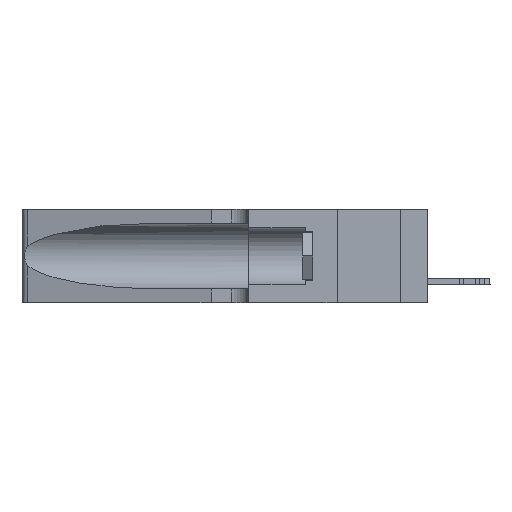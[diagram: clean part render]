
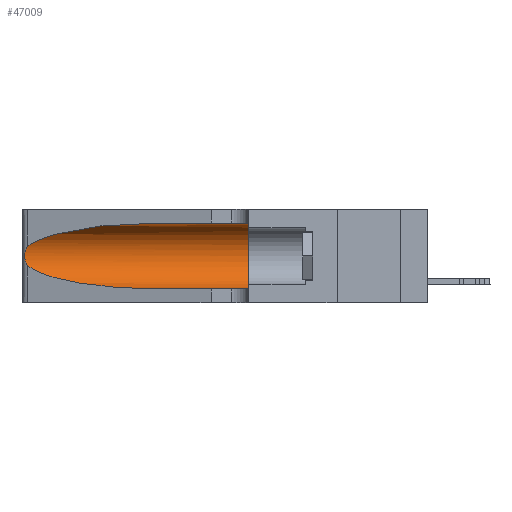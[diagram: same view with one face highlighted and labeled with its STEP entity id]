
A CAD part, left-side view. The second image highlights one B-rep face of the part: STEP entity #47009.
In plain terms, the highlighted cylindrical face has radius 3.308 mm (diameter 6.617 mm), a partial arc.
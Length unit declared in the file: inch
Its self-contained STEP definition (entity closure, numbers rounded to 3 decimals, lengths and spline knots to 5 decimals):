
#547 =( BOUNDED_CURVE ( )  B_SPLINE_CURVE ( 3, ( #36290, #44357, #9405, #29074 ),
 .UNSPECIFIED., .F., .F. ) 
 B_SPLINE_CURVE_WITH_KNOTS ( ( 4, 4 ),
 ( 3.44316, 4.71239 ),
 .UNSPECIFIED. ) 
 CURVE ( )  GEOMETRIC_REPRESENTATION_ITEM ( )  RATIONAL_B_SPLINE_CURVE ( ( 1., 0.87, 0.87, 1. ) ) 
 REPRESENTATION_ITEM ( '' )  );
#750 = EDGE_CURVE ( 'NONE', #4410, #35039, #23873, .T. ) ;
#972 = CARTESIAN_POINT ( 'NONE',  ( 0.25854, 1.2359, 0.20912 ) ) ;
#2075 = CARTESIAN_POINT ( 'NONE',  ( 0.1305, 0.35, 0.185 ) ) ;
#2380 = CARTESIAN_POINT ( 'NONE',  ( 0.25789, 1.23486, 0.15765 ) ) ;
#2528 = EDGE_CURVE ( 'NONE', #36630, #14953, #547, .T. ) ;
#3519 = AXIS2_PLACEMENT_3D ( 'NONE', #8318, #39538, #27631 ) ;
#3695 = LINE ( 'NONE', #27239, #42294 ) ;
#4410 = VERTEX_POINT ( 'NONE', #26532 ) ;
#4888 = CARTESIAN_POINT ( 'NONE',  ( 0.26018, 1.23835, 0.19895 ) ) ;
#4955 = ORIENTED_EDGE ( 'NONE', *, *, #2528, .T. ) ;
#5592 = CARTESIAN_POINT ( 'NONE',  ( 0.25487, 1.22718, 0.14631 ) ) ;
#5952 = CARTESIAN_POINT ( 'NONE',  ( 0.26017, 1.23833, 0.17102 ) ) ;
#7450 = LINE ( 'NONE', #18264, #44226 ) ;
#8318 = CARTESIAN_POINT ( 'NONE',  ( 0.1305, 1.61858, 0.185 ) ) ;
#8747 = CARTESIAN_POINT ( 'NONE',  ( 0.1305, 0.35, 0.05475 ) ) ;
#9405 = CARTESIAN_POINT ( 'NONE',  ( 0.18966, 0.96281, 0.05475 ) ) ;
#10429 = CARTESIAN_POINT ( 'NONE',  ( 0.25487, 1.22718, 0.14631 ) ) ;
#14953 = VERTEX_POINT ( 'NONE', #29104 ) ;
#16022 = ORIENTED_EDGE ( 'NONE', *, *, #750, .T. ) ;
#16343 = CARTESIAN_POINT ( 'NONE',  ( 0.25555, 1.22994, 0.2215 ) ) ;
#16745 = CARTESIAN_POINT ( 'NONE',  ( 0.2373, 1.15595, 0.28018 ) ) ;
#17580 = CARTESIAN_POINT ( 'NONE',  ( 0.1305, 0.35, 0.31525 ) ) ;
#18264 = CARTESIAN_POINT ( 'NONE',  ( 0.1305, 1.61858, 0.05475 ) ) ;
#18874 = EDGE_CURVE ( 'NONE', #14953, #45877, #7450, .T. ) ;
#19837 = CARTESIAN_POINT ( 'NONE',  ( 0.25487, 1.22718, 0.22369 ) ) ;
#19976 = EDGE_CURVE ( 'NONE', #22581, #45877, #32062, .T. ) ;
#20416 = CARTESIAN_POINT ( 'NONE',  ( 0.26075, 1.23896, 0.178 ) ) ;
#21641 = DIRECTION ( 'NONE',  ( 0., -1., 0. ) ) ;
#22538 = AXIS2_PLACEMENT_3D ( 'NONE', #2075, #40370, #29142 ) ;
#22581 = VERTEX_POINT ( 'NONE', #17580 ) ;
#23806 = DIRECTION ( 'NONE',  ( 0., -1., 0. ) ) ;
#23873 =( BOUNDED_CURVE ( )  B_SPLINE_CURVE ( 3, ( #27966, #39545, #16745, #19837 ),
 .UNSPECIFIED., .F., .T. ) 
 B_SPLINE_CURVE_WITH_KNOTS ( ( 4, 4 ),
 ( 1.5708, 2.84003 ),
 .UNSPECIFIED. ) 
 CURVE ( )  GEOMETRIC_REPRESENTATION_ITEM ( )  RATIONAL_B_SPLINE_CURVE ( ( 1., 0.87, 0.87, 1. ) ) 
 REPRESENTATION_ITEM ( '' )  );
#24350 = CARTESIAN_POINT ( 'NONE',  ( 0.26075, 1.23896, 0.19203 ) ) ;
#25482 = B_SPLINE_CURVE_WITH_KNOTS ( 'NONE', 3,
 ( #32424, #16343, #43315, #47317, #972, #4888, #24350, #20416, #5952, #40845, #2380, #36819, #32771, #5592 ),
 .UNSPECIFIED., .F., .F.,
 ( 4, 2, 2, 2, 2, 2, 4 ),
 ( 0., 0.00027, 0.00053, 0.00107, 0.0016, 0.00187, 0.00214 ),
 .UNSPECIFIED. ) ;
#26532 = CARTESIAN_POINT ( 'NONE',  ( 0.1305, 0.72297, 0.31525 ) ) ;
#27239 = CARTESIAN_POINT ( 'NONE',  ( 0.1305, 1.61858, 0.31525 ) ) ;
#27335 = EDGE_CURVE ( 'NONE', #35039, #36630, #25482, .T. ) ;
#27631 = DIRECTION ( 'NONE',  ( 0., 0., -1. ) ) ;
#27966 = CARTESIAN_POINT ( 'NONE',  ( 0.1305, 0.72297, 0.31525 ) ) ;
#29074 = CARTESIAN_POINT ( 'NONE',  ( 0.1305, 0.72297, 0.05475 ) ) ;
#29104 = CARTESIAN_POINT ( 'NONE',  ( 0.1305, 0.72297, 0.05475 ) ) ;
#29142 = DIRECTION ( 'NONE',  ( 0., 0., 1. ) ) ;
#29158 = ORIENTED_EDGE ( 'NONE', *, *, #19976, .F. ) ;
#30181 = CARTESIAN_POINT ( 'NONE',  ( 0.25487, 1.22718, 0.22369 ) ) ;
#31013 = ORIENTED_EDGE ( 'NONE', *, *, #39462, .F. ) ;
#32062 = CIRCLE ( 'NONE', #22538, 0.13025 ) ;
#32424 = CARTESIAN_POINT ( 'NONE',  ( 0.25487, 1.22718, 0.22369 ) ) ;
#32771 = CARTESIAN_POINT ( 'NONE',  ( 0.25555, 1.22993, 0.14849 ) ) ;
#35039 = VERTEX_POINT ( 'NONE', #30181 ) ;
#36290 = CARTESIAN_POINT ( 'NONE',  ( 0.25487, 1.22718, 0.14631 ) ) ;
#36630 = VERTEX_POINT ( 'NONE', #10429 ) ;
#36819 = CARTESIAN_POINT ( 'NONE',  ( 0.25639, 1.23186, 0.15144 ) ) ;
#37402 = CYLINDRICAL_SURFACE ( 'NONE', #3519, 0.13025 ) ;
#38262 = EDGE_LOOP ( 'NONE', ( #16022, #42924, #4955, #46550, #29158, #31013 ) ) ;
#38613 = FACE_OUTER_BOUND ( 'NONE', #38262, .T. ) ;
#39462 = EDGE_CURVE ( 'NONE', #4410, #22581, #3695, .T. ) ;
#39538 = DIRECTION ( 'NONE',  ( 0., -1., 0. ) ) ;
#39545 = CARTESIAN_POINT ( 'NONE',  ( 0.18966, 0.96281, 0.31525 ) ) ;
#40370 = DIRECTION ( 'NONE',  ( 0., 1., 0. ) ) ;
#40845 = CARTESIAN_POINT ( 'NONE',  ( 0.25856, 1.23593, 0.16098 ) ) ;
#42294 = VECTOR ( 'NONE', #23806, 39.37008 ) ;
#42924 = ORIENTED_EDGE ( 'NONE', *, *, #27335, .T. ) ;
#43315 = CARTESIAN_POINT ( 'NONE',  ( 0.25639, 1.23184, 0.21858 ) ) ;
#44226 = VECTOR ( 'NONE', #21641, 39.37008 ) ;
#44357 = CARTESIAN_POINT ( 'NONE',  ( 0.2373, 1.15595, 0.08982 ) ) ;
#45877 = VERTEX_POINT ( 'NONE', #8747 ) ;
#46550 = ORIENTED_EDGE ( 'NONE', *, *, #18874, .T. ) ;
#47009 = ADVANCED_FACE ( 'NONE', ( #38613 ), #37402, .F. ) ;
#47317 = CARTESIAN_POINT ( 'NONE',  ( 0.25787, 1.23484, 0.2124 ) ) ;
